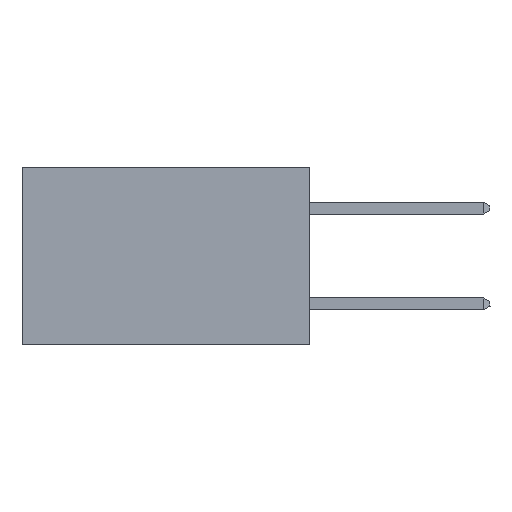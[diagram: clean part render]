
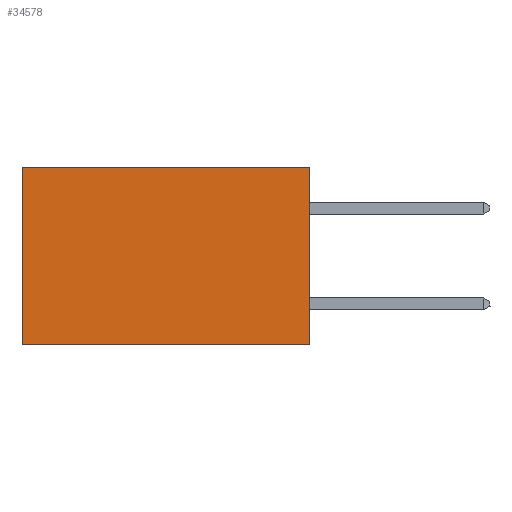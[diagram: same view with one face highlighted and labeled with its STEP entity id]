
A CAD part, left-side view. The second image highlights one B-rep face of the part: STEP entity #34578.
In plain terms, the highlighted planar face has unit normal (-1, 0, 0).
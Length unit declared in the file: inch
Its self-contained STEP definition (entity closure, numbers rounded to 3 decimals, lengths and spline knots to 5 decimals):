
#17 = ORIENTED_EDGE ( 'NONE', *, *, #31580, .T. ) ;
#610 = DIRECTION ( 'NONE',  ( 0., 0., -1. ) ) ;
#763 = CARTESIAN_POINT ( 'NONE',  ( 0.2875, 0.6, 0. ) ) ;
#2330 = CARTESIAN_POINT ( 'NONE',  ( 0.2875, 0., 0. ) ) ;
#6174 = EDGE_CURVE ( 'NONE', #18946, #19738, #31380, .T. ) ;
#6236 = EDGE_LOOP ( 'NONE', ( #17, #8826, #38883, #39471 ) ) ;
#7634 = CARTESIAN_POINT ( 'NONE',  ( 0.2875, 0., 0. ) ) ;
#8826 = ORIENTED_EDGE ( 'NONE', *, *, #6174, .F. ) ;
#8830 = AXIS2_PLACEMENT_3D ( 'NONE', #2330, #35754, #15855 ) ;
#12380 = FACE_OUTER_BOUND ( 'NONE', #6236, .T. ) ;
#12529 = PLANE ( 'NONE',  #8830 ) ;
#13237 = CARTESIAN_POINT ( 'NONE',  ( 0.2875, 0., -0.37 ) ) ;
#14189 = VECTOR ( 'NONE', #18582, 39.37008 ) ;
#15726 = LINE ( 'NONE', #7634, #31324 ) ;
#15855 = DIRECTION ( 'NONE',  ( 0., 0., -1. ) ) ;
#18582 = DIRECTION ( 'NONE',  ( 0., 1., 0. ) ) ;
#18946 = VERTEX_POINT ( 'NONE', #33710 ) ;
#19635 = VERTEX_POINT ( 'NONE', #27881 ) ;
#19738 = VERTEX_POINT ( 'NONE', #38107 ) ;
#20271 = CARTESIAN_POINT ( 'NONE',  ( 0.2875, 0.6, 0. ) ) ;
#25256 = EDGE_CURVE ( 'NONE', #19635, #32160, #40600, .T. ) ;
#27881 = CARTESIAN_POINT ( 'NONE',  ( 0.2875, 0., 0. ) ) ;
#31324 = VECTOR ( 'NONE', #40698, 39.37008 ) ;
#31380 = LINE ( 'NONE', #13237, #32435 ) ;
#31580 = EDGE_CURVE ( 'NONE', #32160, #19738, #34993, .T. ) ;
#32160 = VERTEX_POINT ( 'NONE', #20271 ) ;
#32435 = VECTOR ( 'NONE', #33149, 39.37008 ) ;
#33149 = DIRECTION ( 'NONE',  ( 0., 1., 0. ) ) ;
#33710 = CARTESIAN_POINT ( 'NONE',  ( 0.2875, 0., -0.37 ) ) ;
#34578 = ADVANCED_FACE ( 'NONE', ( #12380 ), #12529, .F. ) ;
#34993 = LINE ( 'NONE', #763, #36037 ) ;
#35126 = CARTESIAN_POINT ( 'NONE',  ( 0.2875, 0., 0. ) ) ;
#35754 = DIRECTION ( 'NONE',  ( 1., 0., 0. ) ) ;
#36037 = VECTOR ( 'NONE', #610, 39.37008 ) ;
#38107 = CARTESIAN_POINT ( 'NONE',  ( 0.2875, 0.6, -0.37 ) ) ;
#38883 = ORIENTED_EDGE ( 'NONE', *, *, #41555, .F. ) ;
#39471 = ORIENTED_EDGE ( 'NONE', *, *, #25256, .T. ) ;
#40600 = LINE ( 'NONE', #35126, #14189 ) ;
#40698 = DIRECTION ( 'NONE',  ( 0., 0., -1. ) ) ;
#41555 = EDGE_CURVE ( 'NONE', #19635, #18946, #15726, .T. ) ;
